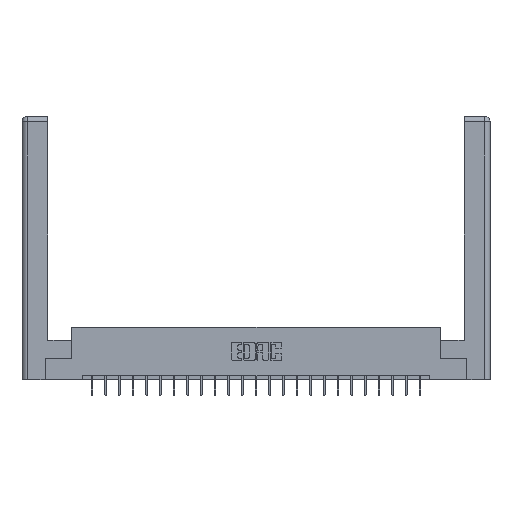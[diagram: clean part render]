
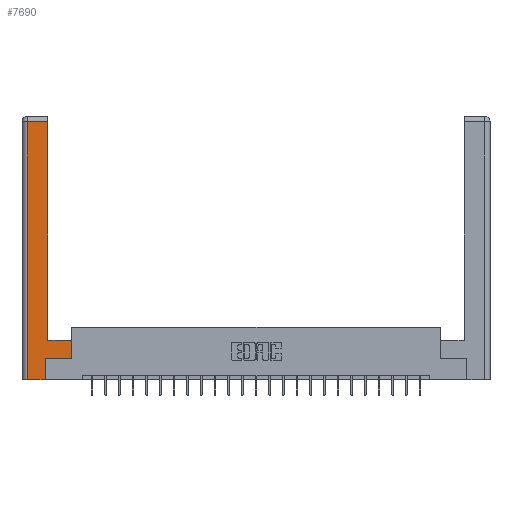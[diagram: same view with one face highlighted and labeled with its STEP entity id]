
A CAD part, top view. The second image highlights one B-rep face of the part: STEP entity #7690.
In plain terms, the highlighted planar face has unit normal (0, 0, 1).
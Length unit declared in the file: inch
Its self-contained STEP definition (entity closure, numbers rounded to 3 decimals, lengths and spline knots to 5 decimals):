
#550 = CARTESIAN_POINT ( 'NONE',  ( 0.0615, 2.94, 0. ) ) ;
#712 = ORIENTED_EDGE ( 'NONE', *, *, #22274, .T. ) ;
#893 = DIRECTION ( 'NONE',  ( 0., 1., 0. ) ) ;
#2038 = DIRECTION ( 'NONE',  ( -1., 0., 0. ) ) ;
#2910 = LINE ( 'NONE', #18543, #17319 ) ;
#3403 = LINE ( 'NONE', #550, #17792 ) ;
#4893 = ORIENTED_EDGE ( 'NONE', *, *, #20881, .T. ) ;
#4958 = CARTESIAN_POINT ( 'NONE',  ( 0.0615, 0., 0. ) ) ;
#5060 = ORIENTED_EDGE ( 'NONE', *, *, #18590, .T. ) ;
#5402 = LINE ( 'NONE', #12898, #23585 ) ;
#5877 = VERTEX_POINT ( 'NONE', #8421 ) ;
#6159 = EDGE_CURVE ( 'NONE', #11736, #6781, #24272, .T. ) ;
#6386 = CARTESIAN_POINT ( 'NONE',  ( 0.295, 2.94, 0. ) ) ;
#6781 = VERTEX_POINT ( 'NONE', #18621 ) ;
#6906 = FACE_OUTER_BOUND ( 'NONE', #8846, .T. ) ;
#6950 = EDGE_CURVE ( 'NONE', #5877, #21932, #19287, .T. ) ;
#7690 = ADVANCED_FACE ( 'NONE', ( #6906 ), #18299, .F. ) ;
#8044 = ORIENTED_EDGE ( 'NONE', *, *, #6950, .T. ) ;
#8378 = EDGE_CURVE ( 'NONE', #6781, #5877, #5402, .T. ) ;
#8421 = CARTESIAN_POINT ( 'NONE',  ( 0.565, 0.45, 0. ) ) ;
#8639 = VERTEX_POINT ( 'NONE', #6386 ) ;
#8846 = EDGE_LOOP ( 'NONE', ( #11378, #4893, #5060, #18148, #712, #23651, #14596, #8044 ) ) ;
#9116 = VERTEX_POINT ( 'NONE', #22858 ) ;
#9367 = EDGE_CURVE ( 'NONE', #22924, #18326, #15817, .T. ) ;
#9699 = CARTESIAN_POINT ( 'NONE',  ( 0.295, 0.45, 0. ) ) ;
#10289 = CARTESIAN_POINT ( 'NONE',  ( 0.265, 0.245, 0. ) ) ;
#10517 = VECTOR ( 'NONE', #893, 39.37008 ) ;
#10781 = EDGE_CURVE ( 'NONE', #21932, #8639, #23801, .T. ) ;
#10883 = DIRECTION ( 'NONE',  ( -1., 0., 0. ) ) ;
#11378 = ORIENTED_EDGE ( 'NONE', *, *, #10781, .T. ) ;
#11447 = CARTESIAN_POINT ( 'NONE',  ( 0.295, 0.45, 0. ) ) ;
#11736 = VERTEX_POINT ( 'NONE', #17424 ) ;
#12898 = CARTESIAN_POINT ( 'NONE',  ( 0.565, 0.45, 0. ) ) ;
#14278 = VECTOR ( 'NONE', #20287, 39.37008 ) ;
#14596 = ORIENTED_EDGE ( 'NONE', *, *, #8378, .T. ) ;
#15611 = AXIS2_PLACEMENT_3D ( 'NONE', #20183, #16095, #10883 ) ;
#15801 = VECTOR ( 'NONE', #23169, 39.37008 ) ;
#15817 = LINE ( 'NONE', #15862, #15801 ) ;
#15862 = CARTESIAN_POINT ( 'NONE',  ( 0.265, 0., 0. ) ) ;
#16095 = DIRECTION ( 'NONE',  ( 0., 0., -1. ) ) ;
#16169 = CARTESIAN_POINT ( 'NONE',  ( 0.265, 0., 0. ) ) ;
#16661 = DIRECTION ( 'NONE',  ( 0., -1., 0. ) ) ;
#16769 = VECTOR ( 'NONE', #18612, 39.37008 ) ;
#17319 = VECTOR ( 'NONE', #16661, 39.37008 ) ;
#17424 = CARTESIAN_POINT ( 'NONE',  ( 0.265, 0.245, 0. ) ) ;
#17792 = VECTOR ( 'NONE', #21129, 39.37008 ) ;
#18148 = ORIENTED_EDGE ( 'NONE', *, *, #9367, .T. ) ;
#18299 = PLANE ( 'NONE',  #15611 ) ;
#18326 = VERTEX_POINT ( 'NONE', #16169 ) ;
#18543 = CARTESIAN_POINT ( 'NONE',  ( 0.0615, 0., 0. ) ) ;
#18590 = EDGE_CURVE ( 'NONE', #9116, #22924, #2910, .T. ) ;
#18612 = DIRECTION ( 'NONE',  ( 0., 1., 0. ) ) ;
#18621 = CARTESIAN_POINT ( 'NONE',  ( 0.565, 0.245, 0. ) ) ;
#19287 = LINE ( 'NONE', #9699, #21921 ) ;
#20183 = CARTESIAN_POINT ( 'NONE',  ( 0., 0., 0. ) ) ;
#20287 = DIRECTION ( 'NONE',  ( 1., 0., 0. ) ) ;
#20330 = CARTESIAN_POINT ( 'NONE',  ( 0.295, 3., 0. ) ) ;
#20881 = EDGE_CURVE ( 'NONE', #8639, #9116, #3403, .T. ) ;
#21129 = DIRECTION ( 'NONE',  ( -1., 0., 0. ) ) ;
#21632 = LINE ( 'NONE', #10289, #10517 ) ;
#21921 = VECTOR ( 'NONE', #2038, 39.37008 ) ;
#21932 = VERTEX_POINT ( 'NONE', #11447 ) ;
#22274 = EDGE_CURVE ( 'NONE', #18326, #11736, #21632, .T. ) ;
#22858 = CARTESIAN_POINT ( 'NONE',  ( 0.0615, 2.94, 0. ) ) ;
#22924 = VERTEX_POINT ( 'NONE', #4958 ) ;
#23169 = DIRECTION ( 'NONE',  ( 1., 0., 0. ) ) ;
#23585 = VECTOR ( 'NONE', #24030, 39.37008 ) ;
#23651 = ORIENTED_EDGE ( 'NONE', *, *, #6159, .T. ) ;
#23801 = LINE ( 'NONE', #20330, #16769 ) ;
#24030 = DIRECTION ( 'NONE',  ( 0., 1., 0. ) ) ;
#24154 = CARTESIAN_POINT ( 'NONE',  ( 0.565, 0.245, 0. ) ) ;
#24272 = LINE ( 'NONE', #24154, #14278 ) ;
